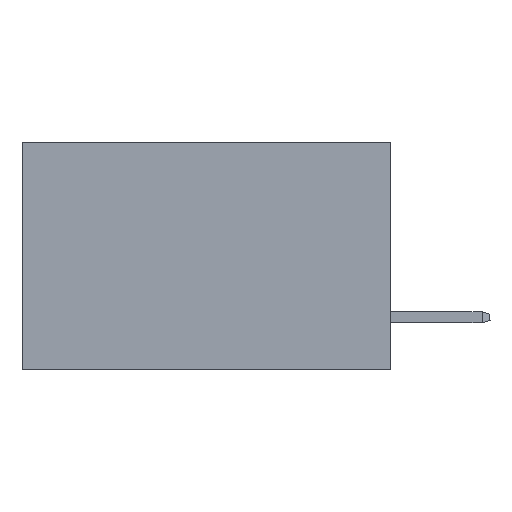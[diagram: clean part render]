
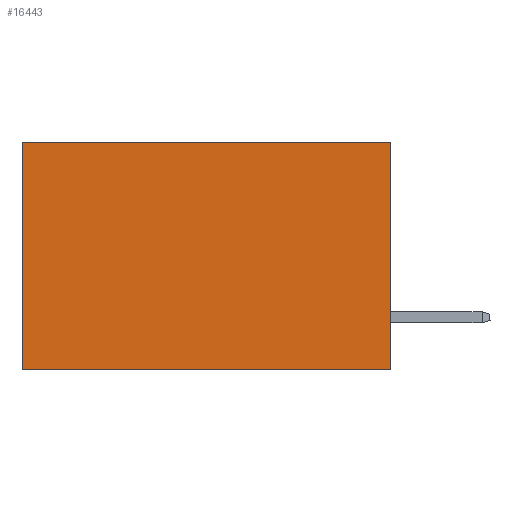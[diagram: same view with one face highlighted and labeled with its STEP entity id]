
A CAD part, left-side view. The second image highlights one B-rep face of the part: STEP entity #16443.
In plain terms, the highlighted planar face has unit normal (-1, 0, 0).
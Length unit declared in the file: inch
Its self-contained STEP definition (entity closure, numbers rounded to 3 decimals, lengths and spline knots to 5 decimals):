
#337 = FACE_OUTER_BOUND ( 'NONE', #12244, .T. ) ;
#3229 = PLANE ( 'NONE',  #31100 ) ;
#3902 = CARTESIAN_POINT ( 'NONE',  ( 0.2875, 0.6, -0.37 ) ) ;
#8622 = VECTOR ( 'NONE', #24383, 39.37008 ) ;
#9234 = VERTEX_POINT ( 'NONE', #37566 ) ;
#10335 = DIRECTION ( 'NONE',  ( 0., 1., 0. ) ) ;
#11780 = VECTOR ( 'NONE', #33593, 39.37008 ) ;
#12244 = EDGE_LOOP ( 'NONE', ( #35592, #34461, #46403, #21403 ) ) ;
#13046 = CARTESIAN_POINT ( 'NONE',  ( 0.2875, 0., 0. ) ) ;
#13764 = LINE ( 'NONE', #17008, #8622 ) ;
#14163 = DIRECTION ( 'NONE',  ( 1., 0., 0. ) ) ;
#14736 = VECTOR ( 'NONE', #10335, 39.37008 ) ;
#16443 = ADVANCED_FACE ( 'NONE', ( #337 ), #3229, .F. ) ;
#16858 = CARTESIAN_POINT ( 'NONE',  ( 0.2875, 0., -0.37 ) ) ;
#17008 = CARTESIAN_POINT ( 'NONE',  ( 0.2875, 0.6, 0. ) ) ;
#17063 = CARTESIAN_POINT ( 'NONE',  ( 0.2875, 0., 0. ) ) ;
#19417 = CARTESIAN_POINT ( 'NONE',  ( 0.2875, 0., 0. ) ) ;
#21403 = ORIENTED_EDGE ( 'NONE', *, *, #43320, .T. ) ;
#21807 = EDGE_CURVE ( 'NONE', #24382, #25542, #41867, .T. ) ;
#23433 = EDGE_CURVE ( 'NONE', #25542, #27806, #30863, .T. ) ;
#24382 = VERTEX_POINT ( 'NONE', #13046 ) ;
#24383 = DIRECTION ( 'NONE',  ( 0., 0., -1. ) ) ;
#25004 = CARTESIAN_POINT ( 'NONE',  ( 0.2875, 0., 0. ) ) ;
#25542 = VERTEX_POINT ( 'NONE', #16858 ) ;
#27575 = CARTESIAN_POINT ( 'NONE',  ( 0.2875, 0., -0.37 ) ) ;
#27806 = VERTEX_POINT ( 'NONE', #3902 ) ;
#28453 = DIRECTION ( 'NONE',  ( 0., 0., -1. ) ) ;
#30863 = LINE ( 'NONE', #27575, #46842 ) ;
#31100 = AXIS2_PLACEMENT_3D ( 'NONE', #25004, #14163, #28453 ) ;
#33593 = DIRECTION ( 'NONE',  ( 0., 0., -1. ) ) ;
#34461 = ORIENTED_EDGE ( 'NONE', *, *, #23433, .F. ) ;
#35245 = EDGE_CURVE ( 'NONE', #9234, #27806, #13764, .T. ) ;
#35592 = ORIENTED_EDGE ( 'NONE', *, *, #35245, .T. ) ;
#37566 = CARTESIAN_POINT ( 'NONE',  ( 0.2875, 0.6, 0. ) ) ;
#38641 = LINE ( 'NONE', #17063, #14736 ) ;
#41867 = LINE ( 'NONE', #19417, #11780 ) ;
#41997 = DIRECTION ( 'NONE',  ( 0., 1., 0. ) ) ;
#43320 = EDGE_CURVE ( 'NONE', #24382, #9234, #38641, .T. ) ;
#46403 = ORIENTED_EDGE ( 'NONE', *, *, #21807, .F. ) ;
#46842 = VECTOR ( 'NONE', #41997, 39.37008 ) ;
